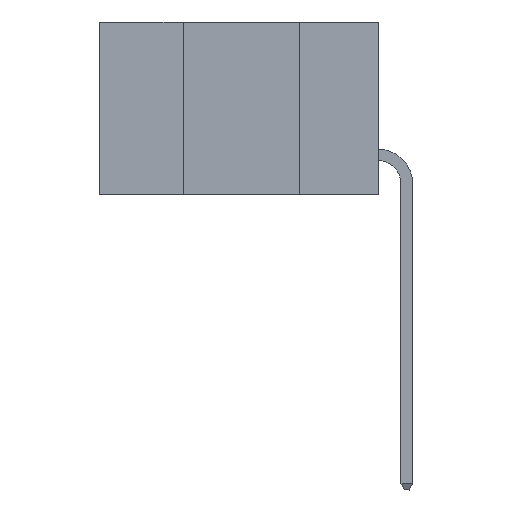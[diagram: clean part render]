
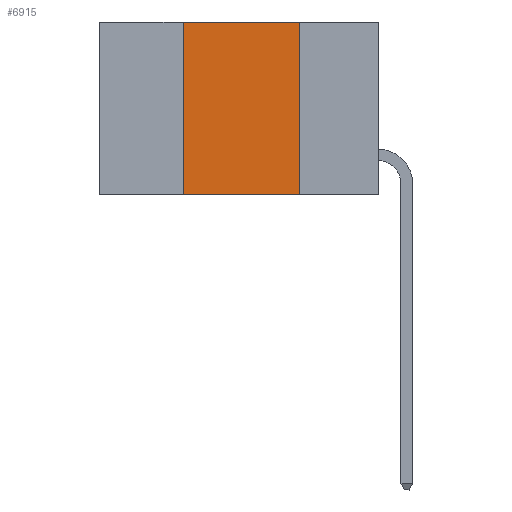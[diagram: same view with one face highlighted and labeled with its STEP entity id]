
A CAD part, left-side view. The second image highlights one B-rep face of the part: STEP entity #6915.
In plain terms, the highlighted planar face has unit normal (-1, 0, 0).
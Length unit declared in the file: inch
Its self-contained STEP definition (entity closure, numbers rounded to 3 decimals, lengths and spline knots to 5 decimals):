
#26 = DIRECTION ( 'NONE',  ( 0., 0., 1. ) ) ;
#69 = FACE_OUTER_BOUND ( 'NONE', #12536, .T. ) ;
#263 = ORIENTED_EDGE ( 'NONE', *, *, #2170, .T. ) ;
#355 = VERTEX_POINT ( 'NONE', #8100 ) ;
#1269 = VECTOR ( 'NONE', #3199, 39.37008 ) ;
#1296 = VECTOR ( 'NONE', #26, 39.37008 ) ;
#1950 = CARTESIAN_POINT ( 'NONE',  ( 0., 0.17, 0. ) ) ;
#2054 = PLANE ( 'NONE',  #14887 ) ;
#2170 = EDGE_CURVE ( 'NONE', #355, #14479, #2504, .T. ) ;
#2314 = VERTEX_POINT ( 'NONE', #8637 ) ;
#2504 = LINE ( 'NONE', #13352, #12036 ) ;
#3012 = EDGE_CURVE ( 'NONE', #355, #2314, #11259, .T. ) ;
#3199 = DIRECTION ( 'NONE',  ( 0., 0., -1. ) ) ;
#3302 = DIRECTION ( 'NONE',  ( 0., 0., -1. ) ) ;
#3448 = VERTEX_POINT ( 'NONE', #12203 ) ;
#3836 = EDGE_CURVE ( 'NONE', #3448, #14479, #11228, .T. ) ;
#5042 = LINE ( 'NONE', #11972, #14574 ) ;
#5669 = ORIENTED_EDGE ( 'NONE', *, *, #3836, .F. ) ;
#6915 = ADVANCED_FACE ( 'NONE', ( #69 ), #2054, .F. ) ;
#8100 = CARTESIAN_POINT ( 'NONE',  ( 0., 0.42, -0.37 ) ) ;
#8321 = CARTESIAN_POINT ( 'NONE',  ( 0., 0.6, 0. ) ) ;
#8637 = CARTESIAN_POINT ( 'NONE',  ( 0., 0.42, 0. ) ) ;
#8822 = EDGE_CURVE ( 'NONE', #2314, #3448, #5042, .T. ) ;
#10801 = DIRECTION ( 'NONE',  ( 1., 0., 0. ) ) ;
#11047 = ORIENTED_EDGE ( 'NONE', *, *, #8822, .F. ) ;
#11228 = LINE ( 'NONE', #1950, #1269 ) ;
#11259 = LINE ( 'NONE', #14902, #1296 ) ;
#11972 = CARTESIAN_POINT ( 'NONE',  ( 0., 0.6, 0. ) ) ;
#12036 = VECTOR ( 'NONE', #14604, 39.37008 ) ;
#12150 = ORIENTED_EDGE ( 'NONE', *, *, #3012, .F. ) ;
#12203 = CARTESIAN_POINT ( 'NONE',  ( 0., 0.17, 0. ) ) ;
#12536 = EDGE_LOOP ( 'NONE', ( #5669, #11047, #12150, #263 ) ) ;
#13200 = DIRECTION ( 'NONE',  ( 0., -1., 0. ) ) ;
#13226 = CARTESIAN_POINT ( 'NONE',  ( 0., 0.17, -0.37 ) ) ;
#13352 = CARTESIAN_POINT ( 'NONE',  ( 0., 0.6, -0.37 ) ) ;
#14479 = VERTEX_POINT ( 'NONE', #13226 ) ;
#14574 = VECTOR ( 'NONE', #13200, 39.37008 ) ;
#14604 = DIRECTION ( 'NONE',  ( 0., -1., 0. ) ) ;
#14887 = AXIS2_PLACEMENT_3D ( 'NONE', #8321, #10801, #3302 ) ;
#14902 = CARTESIAN_POINT ( 'NONE',  ( 0., 0.42, 0. ) ) ;
